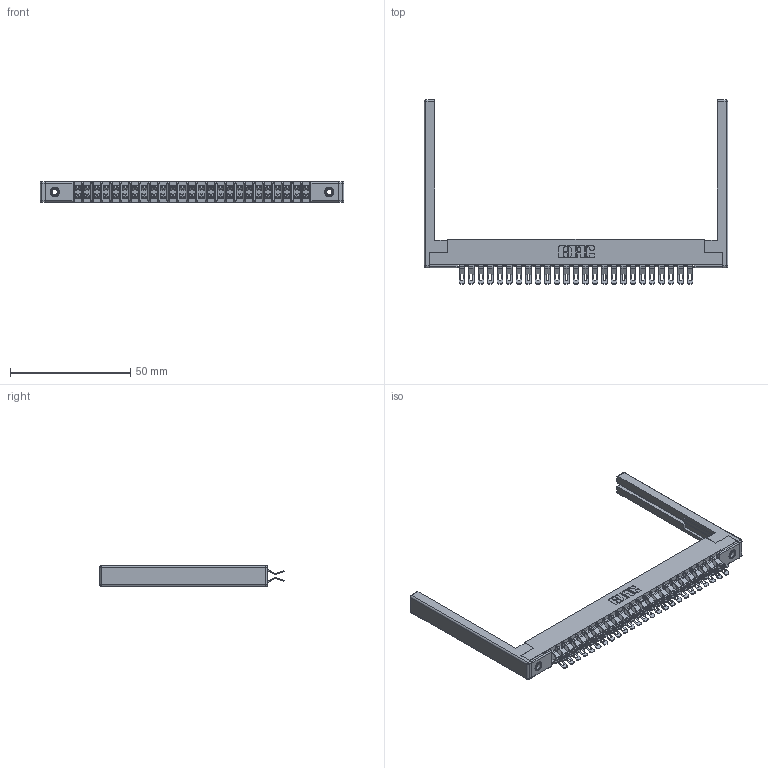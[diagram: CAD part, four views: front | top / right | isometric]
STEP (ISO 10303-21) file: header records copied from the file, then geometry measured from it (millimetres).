
FILE_DESCRIPTION (( 'STEP AP203' ), '1' );
FILE_NAME ('307-050-555-268.STEP', '2019-09-06T11:16:51', ( '' ), ( '' ), 'SwSTEP 2.0', 'SolidWorks 2016', '' );
FILE_SCHEMA (( 'CONFIG_CONTROL_DESIGN' ));
Length unit declared in the file: inch
Products named in the file (5): 307-220-068; 307 Part_.156 Dia Mounting Holes; 307-290-001_555; 307-050-555-268; 345-250-001_345-250-001-102
Assembly tree (55 placements, depth 2):
  307-050-555-268
    307 Part_.156 Dia Mounting Holes
    307-290-001_555  x50
    307-220-068  x2
    345-250-001_345-250-001-102  x2
Bounding box: 126.49 x 76.71 x 8.71 mm (x, y, z)
Volume: 12984 mm3; surface area: 19899.4 mm2
Topology: 55 solids, 55 shells, 3348 faces, 9763 edges, 6350 vertices
Faces by surface type: plane 1858, cylinder 1414, sphere 60, cone 12, torus 4
Entity records: 27624 total; most frequent: CARTESIAN_POINT 4506, ORIENTED_EDGE 4458, DIRECTION 4443, EDGE_CURVE 2229, LINE 1689, VECTOR 1689, VERTEX_POINT 1440, AXIS2_PLACEMENT_3D 1377
